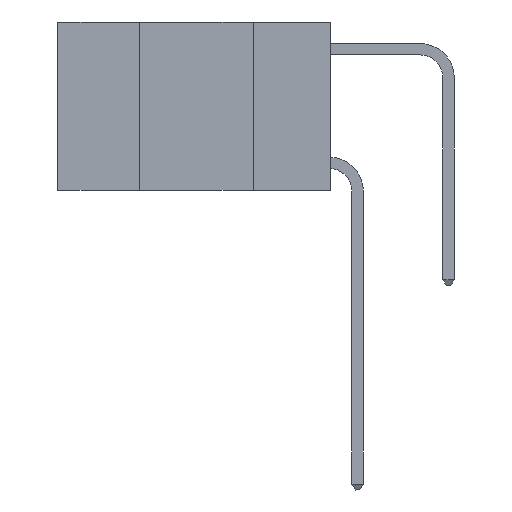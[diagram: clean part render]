
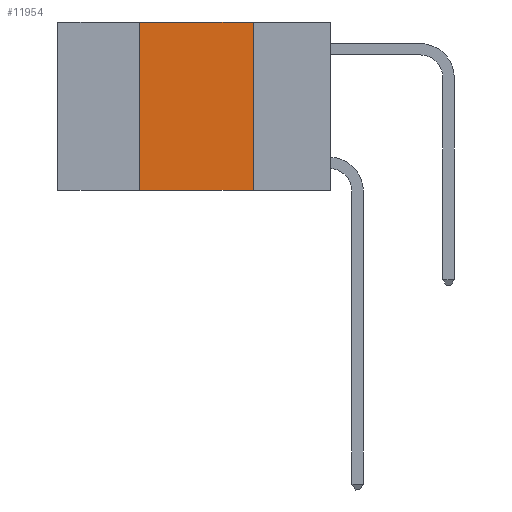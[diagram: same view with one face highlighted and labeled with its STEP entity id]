
A CAD part, left-side view. The second image highlights one B-rep face of the part: STEP entity #11954.
In plain terms, the highlighted planar face has unit normal (-1, 0, 0).
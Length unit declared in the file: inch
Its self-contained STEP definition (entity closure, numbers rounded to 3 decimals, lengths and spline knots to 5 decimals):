
#71 = VERTEX_POINT ( 'NONE', #1676 ) ;
#161 = VECTOR ( 'NONE', #8138, 39.37008 ) ;
#410 = EDGE_CURVE ( 'NONE', #11798, #8709, #11294, .T. ) ;
#749 = CARTESIAN_POINT ( 'NONE',  ( 0., 0.6, 0. ) ) ;
#887 = FACE_OUTER_BOUND ( 'NONE', #5450, .T. ) ;
#1351 = ORIENTED_EDGE ( 'NONE', *, *, #5776, .F. ) ;
#1676 = CARTESIAN_POINT ( 'NONE',  ( 0., 0.42, 0. ) ) ;
#2273 = CARTESIAN_POINT ( 'NONE',  ( 0., 0.17, 0. ) ) ;
#3030 = VERTEX_POINT ( 'NONE', #2273 ) ;
#3035 = LINE ( 'NONE', #8996, #161 ) ;
#3300 = DIRECTION ( 'NONE',  ( 0., -1., 0. ) ) ;
#3484 = DIRECTION ( 'NONE',  ( 0., -1., 0. ) ) ;
#3974 = LINE ( 'NONE', #7810, #11889 ) ;
#4178 = ORIENTED_EDGE ( 'NONE', *, *, #11107, .F. ) ;
#4680 = DIRECTION ( 'NONE',  ( 1., 0., 0. ) ) ;
#4819 = PLANE ( 'NONE',  #9938 ) ;
#5450 = EDGE_LOOP ( 'NONE', ( #4178, #1351, #11381, #10702 ) ) ;
#5776 = EDGE_CURVE ( 'NONE', #71, #3030, #7365, .T. ) ;
#6444 = CARTESIAN_POINT ( 'NONE',  ( 0., 0.6, 0. ) ) ;
#7071 = CARTESIAN_POINT ( 'NONE',  ( 0., 0.17, -0.37 ) ) ;
#7189 = CARTESIAN_POINT ( 'NONE',  ( 0., 0.6, -0.37 ) ) ;
#7363 = VECTOR ( 'NONE', #3300, 39.37008 ) ;
#7365 = LINE ( 'NONE', #6444, #8975 ) ;
#7810 = CARTESIAN_POINT ( 'NONE',  ( 0., 0.17, 0. ) ) ;
#7824 = EDGE_CURVE ( 'NONE', #11798, #71, #3035, .T. ) ;
#8138 = DIRECTION ( 'NONE',  ( 0., 0., 1. ) ) ;
#8599 = DIRECTION ( 'NONE',  ( 0., 0., -1. ) ) ;
#8709 = VERTEX_POINT ( 'NONE', #7071 ) ;
#8975 = VECTOR ( 'NONE', #3484, 39.37008 ) ;
#8996 = CARTESIAN_POINT ( 'NONE',  ( 0., 0.42, 0. ) ) ;
#9683 = CARTESIAN_POINT ( 'NONE',  ( 0., 0.42, -0.37 ) ) ;
#9938 = AXIS2_PLACEMENT_3D ( 'NONE', #749, #4680, #8599 ) ;
#10702 = ORIENTED_EDGE ( 'NONE', *, *, #410, .T. ) ;
#11107 = EDGE_CURVE ( 'NONE', #3030, #8709, #3974, .T. ) ;
#11294 = LINE ( 'NONE', #7189, #7363 ) ;
#11381 = ORIENTED_EDGE ( 'NONE', *, *, #7824, .F. ) ;
#11798 = VERTEX_POINT ( 'NONE', #9683 ) ;
#11889 = VECTOR ( 'NONE', #12519, 39.37008 ) ;
#11954 = ADVANCED_FACE ( 'NONE', ( #887 ), #4819, .F. ) ;
#12519 = DIRECTION ( 'NONE',  ( 0., 0., -1. ) ) ;
